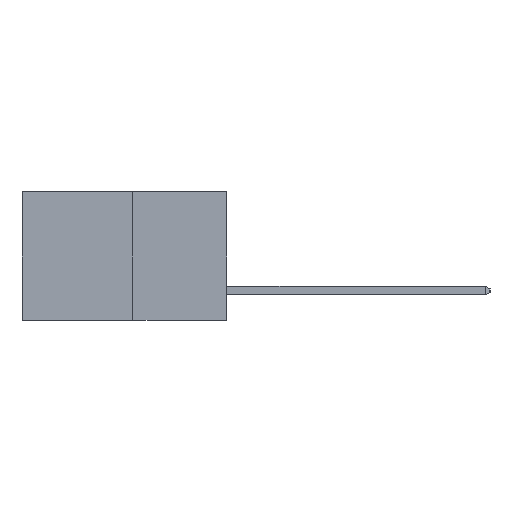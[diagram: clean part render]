
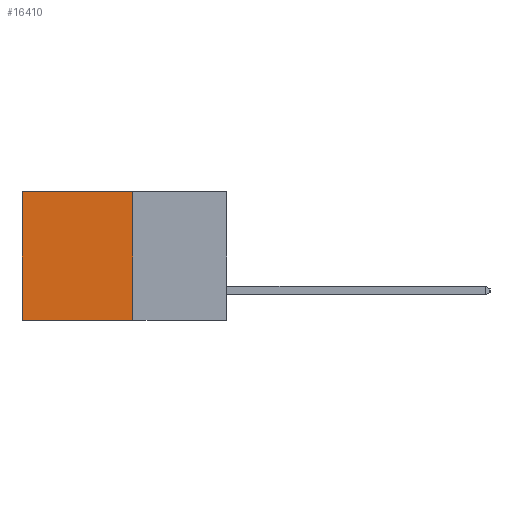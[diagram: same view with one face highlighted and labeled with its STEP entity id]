
A CAD part, left-side view. The second image highlights one B-rep face of the part: STEP entity #16410.
In plain terms, the highlighted planar face has unit normal (-1, 0, 0).
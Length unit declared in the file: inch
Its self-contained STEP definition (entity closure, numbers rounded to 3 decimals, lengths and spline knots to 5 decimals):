
#277 = VECTOR ( 'NONE', #23378, 39.37008 ) ;
#1094 = VECTOR ( 'NONE', #9499, 39.37008 ) ;
#1696 = VERTEX_POINT ( 'NONE', #15558 ) ;
#2215 = ORIENTED_EDGE ( 'NONE', *, *, #8794, .T. ) ;
#4207 = CARTESIAN_POINT ( 'NONE',  ( 0.277, 0.27, -0.37 ) ) ;
#4370 = FACE_OUTER_BOUND ( 'NONE', #8058, .T. ) ;
#4925 = VERTEX_POINT ( 'NONE', #16074 ) ;
#5588 = ORIENTED_EDGE ( 'NONE', *, *, #22832, .T. ) ;
#5716 = LINE ( 'NONE', #13210, #277 ) ;
#6262 = PLANE ( 'NONE',  #22316 ) ;
#6581 = ORIENTED_EDGE ( 'NONE', *, *, #16146, .F. ) ;
#8058 = EDGE_LOOP ( 'NONE', ( #2215, #6581, #17048, #5588 ) ) ;
#8330 = DIRECTION ( 'NONE',  ( 0., 0., -1. ) ) ;
#8794 = EDGE_CURVE ( 'NONE', #9583, #4925, #24111, .T. ) ;
#9499 = DIRECTION ( 'NONE',  ( 0., 1., 0. ) ) ;
#9583 = VERTEX_POINT ( 'NONE', #18083 ) ;
#10187 = VECTOR ( 'NONE', #26005, 39.37008 ) ;
#11241 = CARTESIAN_POINT ( 'NONE',  ( 0.277, 0.59, -0.37 ) ) ;
#12066 = VERTEX_POINT ( 'NONE', #13946 ) ;
#13210 = CARTESIAN_POINT ( 'NONE',  ( 0.277, 0.27, -0.37 ) ) ;
#13227 = VECTOR ( 'NONE', #15342, 39.37008 ) ;
#13946 = CARTESIAN_POINT ( 'NONE',  ( 0.277, 0.27, 0. ) ) ;
#14810 = EDGE_CURVE ( 'NONE', #12066, #1696, #5716, .T. ) ;
#15342 = DIRECTION ( 'NONE',  ( 0., 0., -1. ) ) ;
#15558 = CARTESIAN_POINT ( 'NONE',  ( 0.277, 0.27, -0.37 ) ) ;
#16074 = CARTESIAN_POINT ( 'NONE',  ( 0.277, 0.59, -0.37 ) ) ;
#16142 = LINE ( 'NONE', #21714, #1094 ) ;
#16146 = EDGE_CURVE ( 'NONE', #1696, #4925, #26528, .T. ) ;
#16410 = ADVANCED_FACE ( 'NONE', ( #4370 ), #6262, .F. ) ;
#17048 = ORIENTED_EDGE ( 'NONE', *, *, #14810, .F. ) ;
#18083 = CARTESIAN_POINT ( 'NONE',  ( 0.277, 0.59, 0. ) ) ;
#20547 = DIRECTION ( 'NONE',  ( 1., 0., 0. ) ) ;
#21714 = CARTESIAN_POINT ( 'NONE',  ( 0.277, 0.27, 0. ) ) ;
#22316 = AXIS2_PLACEMENT_3D ( 'NONE', #4207, #20547, #8330 ) ;
#22832 = EDGE_CURVE ( 'NONE', #12066, #9583, #16142, .T. ) ;
#23378 = DIRECTION ( 'NONE',  ( 0., 0., -1. ) ) ;
#23925 = CARTESIAN_POINT ( 'NONE',  ( 0.277, 0.27, -0.37 ) ) ;
#24111 = LINE ( 'NONE', #11241, #13227 ) ;
#26005 = DIRECTION ( 'NONE',  ( 0., 1., 0. ) ) ;
#26528 = LINE ( 'NONE', #23925, #10187 ) ;
